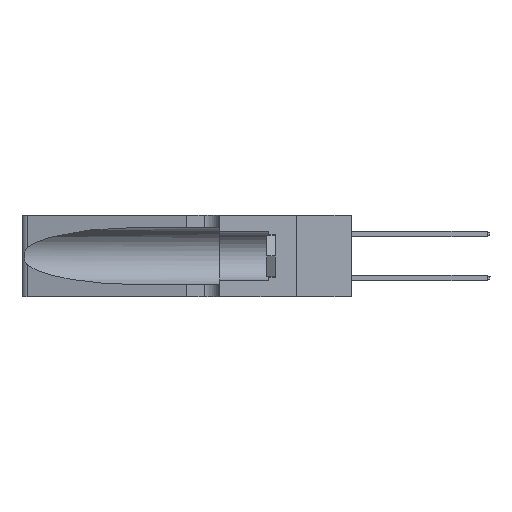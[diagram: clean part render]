
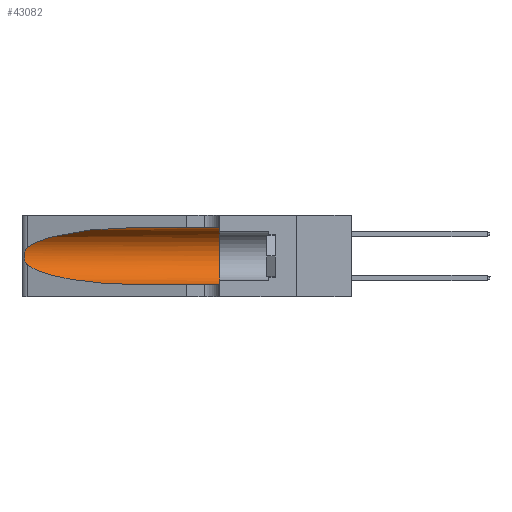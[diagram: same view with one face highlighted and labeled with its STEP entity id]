
A CAD part, left-side view. The second image highlights one B-rep face of the part: STEP entity #43082.
In plain terms, the highlighted cylindrical face has radius 3.308 mm (diameter 6.617 mm), a partial arc.
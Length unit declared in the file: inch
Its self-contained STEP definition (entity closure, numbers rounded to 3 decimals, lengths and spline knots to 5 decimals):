
#1082 = EDGE_CURVE ( 'NONE', #40136, #25320, #46289, .T. ) ;
#1154 = CARTESIAN_POINT ( 'NONE',  ( 0.1305, 0.35, 0.05475 ) ) ;
#1299 =( BOUNDED_CURVE ( )  B_SPLINE_CURVE ( 3, ( #16488, #23703, #8968, #42005 ),
 .UNSPECIFIED., .F., .F. ) 
 B_SPLINE_CURVE_WITH_KNOTS ( ( 4, 4 ),
 ( 1.5708, 2.84003 ),
 .UNSPECIFIED. ) 
 CURVE ( )  GEOMETRIC_REPRESENTATION_ITEM ( )  RATIONAL_B_SPLINE_CURVE ( ( 1., 0.87, 0.87, 1. ) ) 
 REPRESENTATION_ITEM ( '' )  );
#2037 = CARTESIAN_POINT ( 'NONE',  ( 0.26018, 1.23835, 0.19895 ) ) ;
#2510 = CARTESIAN_POINT ( 'NONE',  ( 0.25789, 1.23486, 0.15765 ) ) ;
#2976 = CARTESIAN_POINT ( 'NONE',  ( 0.25639, 1.23186, 0.15144 ) ) ;
#5331 = EDGE_LOOP ( 'NONE', ( #34886, #15623, #44966, #29721, #37668, #36856 ) ) ;
#5911 = CARTESIAN_POINT ( 'NONE',  ( 0.1305, 0.72297, 0.05475 ) ) ;
#8584 = EDGE_CURVE ( 'NONE', #25320, #33570, #23638, .T. ) ;
#8611 = DIRECTION ( 'NONE',  ( 0., -1., 0. ) ) ;
#8878 = AXIS2_PLACEMENT_3D ( 'NONE', #45511, #8611, #23499 ) ;
#8968 = CARTESIAN_POINT ( 'NONE',  ( 0.2373, 1.15595, 0.28018 ) ) ;
#8995 = VERTEX_POINT ( 'NONE', #34953 ) ;
#9073 = CARTESIAN_POINT ( 'NONE',  ( 0.1305, 0.35, 0.185 ) ) ;
#11732 = CYLINDRICAL_SURFACE ( 'NONE', #8878, 0.13025 ) ;
#12717 = VERTEX_POINT ( 'NONE', #41104 ) ;
#12951 = CARTESIAN_POINT ( 'NONE',  ( 0.25487, 1.22718, 0.22369 ) ) ;
#12992 = CARTESIAN_POINT ( 'NONE',  ( 0.25487, 1.22718, 0.14631 ) ) ;
#13271 = CARTESIAN_POINT ( 'NONE',  ( 0.25639, 1.23184, 0.21858 ) ) ;
#14000 = EDGE_CURVE ( 'NONE', #12717, #33570, #35346, .T. ) ;
#14216 = DIRECTION ( 'NONE',  ( 0., -1., 0. ) ) ;
#15623 = ORIENTED_EDGE ( 'NONE', *, *, #25364, .T. ) ;
#16488 = CARTESIAN_POINT ( 'NONE',  ( 0.1305, 0.72297, 0.31525 ) ) ;
#16941 = CARTESIAN_POINT ( 'NONE',  ( 0.26075, 1.23896, 0.19203 ) ) ;
#20635 = CARTESIAN_POINT ( 'NONE',  ( 0.26075, 1.23896, 0.178 ) ) ;
#21419 = CARTESIAN_POINT ( 'NONE',  ( 0.25555, 1.22993, 0.14849 ) ) ;
#21867 = EDGE_CURVE ( 'NONE', #8995, #43195, #1299, .T. ) ;
#22299 = CARTESIAN_POINT ( 'NONE',  ( 0.25487, 1.22718, 0.22369 ) ) ;
#23181 = FACE_OUTER_BOUND ( 'NONE', #5331, .T. ) ;
#23499 = DIRECTION ( 'NONE',  ( 0., 0., -1. ) ) ;
#23638 = LINE ( 'NONE', #40484, #38578 ) ;
#23703 = CARTESIAN_POINT ( 'NONE',  ( 0.18966, 0.96281, 0.31525 ) ) ;
#24172 = EDGE_CURVE ( 'NONE', #8995, #12717, #42326, .T. ) ;
#24197 = B_SPLINE_CURVE_WITH_KNOTS ( 'NONE', 3,
 ( #12951, #39253, #13271, #38933, #46473, #2037, #16941, #20635, #46321, #24456, #2510, #2976, #21419, #46954 ),
 .UNSPECIFIED., .F., .F.,
 ( 4, 2, 2, 2, 2, 2, 4 ),
 ( 0., 0.00027, 0.00053, 0.00107, 0.0016, 0.00187, 0.00214 ),
 .UNSPECIFIED. ) ;
#24456 = CARTESIAN_POINT ( 'NONE',  ( 0.25856, 1.23593, 0.16098 ) ) ;
#25320 = VERTEX_POINT ( 'NONE', #5911 ) ;
#25364 = EDGE_CURVE ( 'NONE', #43195, #40136, #24197, .T. ) ;
#26933 = CARTESIAN_POINT ( 'NONE',  ( 0.2373, 1.15595, 0.08982 ) ) ;
#27838 = CARTESIAN_POINT ( 'NONE',  ( 0.25487, 1.22718, 0.14631 ) ) ;
#29069 = DIRECTION ( 'NONE',  ( 0., -1., 0. ) ) ;
#29721 = ORIENTED_EDGE ( 'NONE', *, *, #8584, .T. ) ;
#32557 = VECTOR ( 'NONE', #14216, 39.37008 ) ;
#33570 = VERTEX_POINT ( 'NONE', #1154 ) ;
#34720 = DIRECTION ( 'NONE',  ( 0., 1., 0. ) ) ;
#34886 = ORIENTED_EDGE ( 'NONE', *, *, #21867, .T. ) ;
#34953 = CARTESIAN_POINT ( 'NONE',  ( 0.1305, 0.72297, 0.31525 ) ) ;
#35346 = CIRCLE ( 'NONE', #42898, 0.13025 ) ;
#36166 = CARTESIAN_POINT ( 'NONE',  ( 0.1305, 1.61858, 0.31525 ) ) ;
#36856 = ORIENTED_EDGE ( 'NONE', *, *, #24172, .F. ) ;
#37668 = ORIENTED_EDGE ( 'NONE', *, *, #14000, .F. ) ;
#38422 = DIRECTION ( 'NONE',  ( 0., 0., 1. ) ) ;
#38578 = VECTOR ( 'NONE', #29069, 39.37008 ) ;
#38660 = CARTESIAN_POINT ( 'NONE',  ( 0.18966, 0.96281, 0.05475 ) ) ;
#38933 = CARTESIAN_POINT ( 'NONE',  ( 0.25787, 1.23484, 0.2124 ) ) ;
#39253 = CARTESIAN_POINT ( 'NONE',  ( 0.25555, 1.22994, 0.2215 ) ) ;
#40136 = VERTEX_POINT ( 'NONE', #27838 ) ;
#40484 = CARTESIAN_POINT ( 'NONE',  ( 0.1305, 1.61858, 0.05475 ) ) ;
#41104 = CARTESIAN_POINT ( 'NONE',  ( 0.1305, 0.35, 0.31525 ) ) ;
#42005 = CARTESIAN_POINT ( 'NONE',  ( 0.25487, 1.22718, 0.22369 ) ) ;
#42326 = LINE ( 'NONE', #36166, #32557 ) ;
#42898 = AXIS2_PLACEMENT_3D ( 'NONE', #9073, #34720, #38422 ) ;
#43082 = ADVANCED_FACE ( 'NONE', ( #23181 ), #11732, .F. ) ;
#43195 = VERTEX_POINT ( 'NONE', #22299 ) ;
#44966 = ORIENTED_EDGE ( 'NONE', *, *, #1082, .T. ) ;
#45511 = CARTESIAN_POINT ( 'NONE',  ( 0.1305, 1.61858, 0.185 ) ) ;
#45893 = CARTESIAN_POINT ( 'NONE',  ( 0.1305, 0.72297, 0.05475 ) ) ;
#46289 =( BOUNDED_CURVE ( )  B_SPLINE_CURVE ( 3, ( #12992, #26933, #38660, #45893 ),
 .UNSPECIFIED., .F., .T. ) 
 B_SPLINE_CURVE_WITH_KNOTS ( ( 4, 4 ),
 ( 3.44316, 4.71239 ),
 .UNSPECIFIED. ) 
 CURVE ( )  GEOMETRIC_REPRESENTATION_ITEM ( )  RATIONAL_B_SPLINE_CURVE ( ( 1., 0.87, 0.87, 1. ) ) 
 REPRESENTATION_ITEM ( '' )  );
#46321 = CARTESIAN_POINT ( 'NONE',  ( 0.26017, 1.23833, 0.17102 ) ) ;
#46473 = CARTESIAN_POINT ( 'NONE',  ( 0.25854, 1.2359, 0.20912 ) ) ;
#46954 = CARTESIAN_POINT ( 'NONE',  ( 0.25487, 1.22718, 0.14631 ) ) ;
